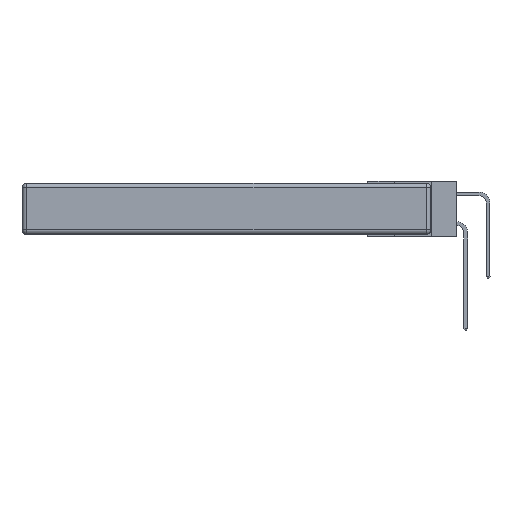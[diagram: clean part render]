
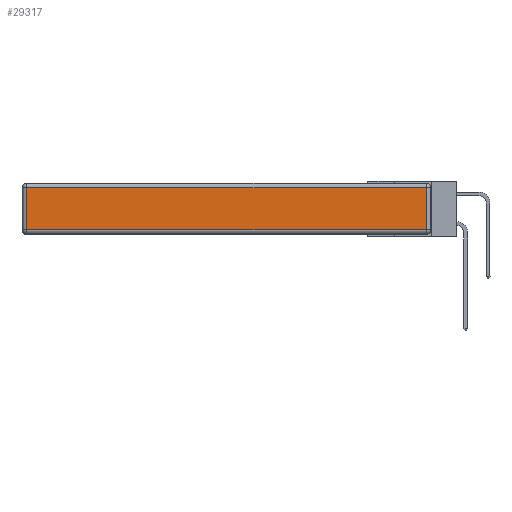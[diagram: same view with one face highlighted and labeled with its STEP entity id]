
A CAD part, left-side view. The second image highlights one B-rep face of the part: STEP entity #29317.
In plain terms, the highlighted planar face has unit normal (-1, 0, 0).
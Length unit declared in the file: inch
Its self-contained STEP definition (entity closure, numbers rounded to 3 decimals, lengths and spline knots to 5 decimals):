
#708 = EDGE_CURVE ( 'NONE', #22030, #19863, #9651, .T. ) ;
#1323 = CARTESIAN_POINT ( 'NONE',  ( 0., 0.03, -0.03 ) ) ;
#1829 = VECTOR ( 'NONE', #11921, 39.37008 ) ;
#2859 = DIRECTION ( 'NONE',  ( -1., 0., 0. ) ) ;
#2954 = LINE ( 'NONE', #9500, #1829 ) ;
#4301 = EDGE_LOOP ( 'NONE', ( #21235, #8663, #26097, #25384 ) ) ;
#4736 = LINE ( 'NONE', #5999, #25946 ) ;
#5999 = CARTESIAN_POINT ( 'NONE',  ( 0., 2.72, -0.343 ) ) ;
#6710 = CARTESIAN_POINT ( 'NONE',  ( 0., 2.72, -0.03 ) ) ;
#8442 = DIRECTION ( 'NONE',  ( 0., 0., -1. ) ) ;
#8627 = EDGE_CURVE ( 'NONE', #30281, #22509, #4736, .T. ) ;
#8663 = ORIENTED_EDGE ( 'NONE', *, *, #708, .T. ) ;
#8896 = VECTOR ( 'NONE', #12789, 39.37008 ) ;
#9500 = CARTESIAN_POINT ( 'NONE',  ( 0., 0., -0.313 ) ) ;
#9651 = LINE ( 'NONE', #17550, #8896 ) ;
#11921 = DIRECTION ( 'NONE',  ( 0., -1., 0. ) ) ;
#12629 = DIRECTION ( 'NONE',  ( 0., 0., 1. ) ) ;
#12789 = DIRECTION ( 'NONE',  ( 0., 0., 1. ) ) ;
#13817 = EDGE_CURVE ( 'NONE', #22509, #22030, #2954, .T. ) ;
#16266 = LINE ( 'NONE', #21508, #28369 ) ;
#16799 = AXIS2_PLACEMENT_3D ( 'NONE', #26894, #2859, #12629 ) ;
#17550 = CARTESIAN_POINT ( 'NONE',  ( 0., 0.03, -0.343 ) ) ;
#19706 = PLANE ( 'NONE',  #16799 ) ;
#19863 = VERTEX_POINT ( 'NONE', #1323 ) ;
#20649 = FACE_OUTER_BOUND ( 'NONE', #4301, .T. ) ;
#21235 = ORIENTED_EDGE ( 'NONE', *, *, #13817, .T. ) ;
#21508 = CARTESIAN_POINT ( 'NONE',  ( 0., 2.75, -0.03 ) ) ;
#22030 = VERTEX_POINT ( 'NONE', #25324 ) ;
#22509 = VERTEX_POINT ( 'NONE', #30001 ) ;
#22911 = EDGE_CURVE ( 'NONE', #19863, #30281, #16266, .T. ) ;
#25324 = CARTESIAN_POINT ( 'NONE',  ( 0., 0.03, -0.313 ) ) ;
#25384 = ORIENTED_EDGE ( 'NONE', *, *, #8627, .T. ) ;
#25946 = VECTOR ( 'NONE', #8442, 39.37008 ) ;
#26097 = ORIENTED_EDGE ( 'NONE', *, *, #22911, .T. ) ;
#26894 = CARTESIAN_POINT ( 'NONE',  ( 0., 0., -0.343 ) ) ;
#28369 = VECTOR ( 'NONE', #28509, 39.37008 ) ;
#28509 = DIRECTION ( 'NONE',  ( 0., 1., 0. ) ) ;
#29317 = ADVANCED_FACE ( 'NONE', ( #20649 ), #19706, .T. ) ;
#30001 = CARTESIAN_POINT ( 'NONE',  ( 0., 2.72, -0.313 ) ) ;
#30281 = VERTEX_POINT ( 'NONE', #6710 ) ;
